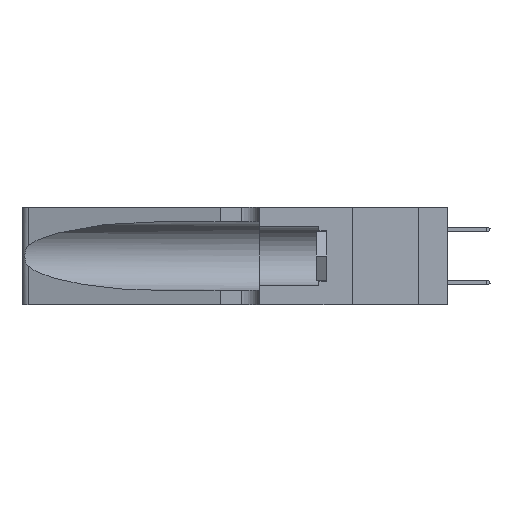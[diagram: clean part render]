
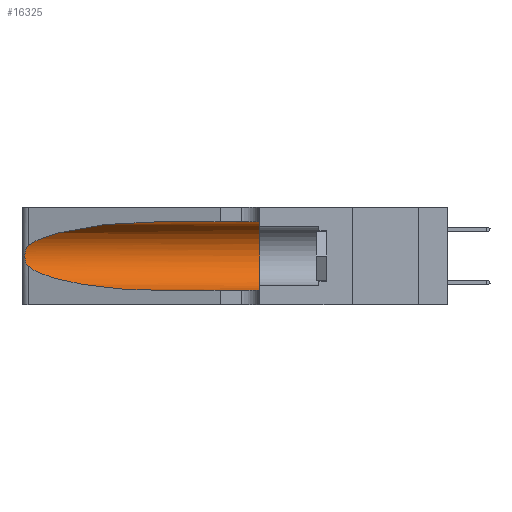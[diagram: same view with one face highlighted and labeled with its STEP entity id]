
A CAD part, left-side view. The second image highlights one B-rep face of the part: STEP entity #16325.
In plain terms, the highlighted cylindrical face has radius 3.308 mm (diameter 6.617 mm), a partial arc.
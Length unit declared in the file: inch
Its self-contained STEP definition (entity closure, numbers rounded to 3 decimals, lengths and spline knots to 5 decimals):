
#43 = CARTESIAN_POINT ( 'NONE',  ( 0.1305, 1.61858, 0.185 ) ) ;
#162 = ORIENTED_EDGE ( 'NONE', *, *, #4983, .F. ) ;
#1116 = CARTESIAN_POINT ( 'NONE',  ( 0.25487, 1.22718, 0.14631 ) ) ;
#1506 = CARTESIAN_POINT ( 'NONE',  ( 0.25555, 1.22994, 0.2215 ) ) ;
#3248 = B_SPLINE_CURVE_WITH_KNOTS ( 'NONE', 3,
 ( #15390, #1506, #21272, #32494, #4783, #7573, #10356, #21038, #30301, #34028, #19004, #22114, #27358, #10735 ),
 .UNSPECIFIED., .F., .F.,
 ( 4, 2, 2, 2, 2, 2, 4 ),
 ( 0., 0.00027, 0.00053, 0.00107, 0.0016, 0.00187, 0.00214 ),
 .UNSPECIFIED. ) ;
#3458 = ORIENTED_EDGE ( 'NONE', *, *, #6924, .T. ) ;
#4783 = CARTESIAN_POINT ( 'NONE',  ( 0.25854, 1.2359, 0.20912 ) ) ;
#4849 = ORIENTED_EDGE ( 'NONE', *, *, #20358, .T. ) ;
#4983 = EDGE_CURVE ( 'NONE', #24811, #6345, #30905, .T. ) ;
#5214 = VERTEX_POINT ( 'NONE', #15593 ) ;
#5854 = DIRECTION ( 'NONE',  ( 0., -1., 0. ) ) ;
#6345 = VERTEX_POINT ( 'NONE', #18593 ) ;
#6441 = VERTEX_POINT ( 'NONE', #10601 ) ;
#6924 = EDGE_CURVE ( 'NONE', #6441, #5214, #16180, .T. ) ;
#7409 = ORIENTED_EDGE ( 'NONE', *, *, #34758, .F. ) ;
#7573 = CARTESIAN_POINT ( 'NONE',  ( 0.26018, 1.23835, 0.19895 ) ) ;
#9037 = LINE ( 'NONE', #17661, #29029 ) ;
#10340 = CARTESIAN_POINT ( 'NONE',  ( 0.2373, 1.15595, 0.08982 ) ) ;
#10356 = CARTESIAN_POINT ( 'NONE',  ( 0.26075, 1.23896, 0.19203 ) ) ;
#10601 = CARTESIAN_POINT ( 'NONE',  ( 0.1305, 0.72297, 0.31525 ) ) ;
#10718 = CARTESIAN_POINT ( 'NONE',  ( 0.25487, 1.22718, 0.14631 ) ) ;
#10735 = CARTESIAN_POINT ( 'NONE',  ( 0.25487, 1.22718, 0.14631 ) ) ;
#11942 = DIRECTION ( 'NONE',  ( 0., -1., 0. ) ) ;
#13049 = CARTESIAN_POINT ( 'NONE',  ( 0.25487, 1.22718, 0.22369 ) ) ;
#13849 = CARTESIAN_POINT ( 'NONE',  ( 0.1305, 0.35, 0.185 ) ) ;
#15390 = CARTESIAN_POINT ( 'NONE',  ( 0.25487, 1.22718, 0.22369 ) ) ;
#15593 = CARTESIAN_POINT ( 'NONE',  ( 0.25487, 1.22718, 0.22369 ) ) ;
#15768 = CARTESIAN_POINT ( 'NONE',  ( 0.1305, 0.35, 0.31525 ) ) ;
#15977 = VERTEX_POINT ( 'NONE', #33857 ) ;
#15984 = FACE_OUTER_BOUND ( 'NONE', #34452, .T. ) ;
#16180 =( BOUNDED_CURVE ( )  B_SPLINE_CURVE ( 3, ( #24587, #35395, #29949, #13049 ),
 .UNSPECIFIED., .F., .F. ) 
 B_SPLINE_CURVE_WITH_KNOTS ( ( 4, 4 ),
 ( 1.5708, 2.84003 ),
 .UNSPECIFIED. ) 
 CURVE ( )  GEOMETRIC_REPRESENTATION_ITEM ( )  RATIONAL_B_SPLINE_CURVE ( ( 1., 0.87, 0.87, 1. ) ) 
 REPRESENTATION_ITEM ( '' )  );
#16193 = CARTESIAN_POINT ( 'NONE',  ( 0.18966, 0.96281, 0.05475 ) ) ;
#16325 = ADVANCED_FACE ( 'NONE', ( #15984 ), #25102, .F. ) ;
#16645 = DIRECTION ( 'NONE',  ( 0., 0., 1. ) ) ;
#17661 = CARTESIAN_POINT ( 'NONE',  ( 0.1305, 1.61858, 0.31525 ) ) ;
#18370 = EDGE_CURVE ( 'NONE', #5214, #28087, #3248, .T. ) ;
#18593 = CARTESIAN_POINT ( 'NONE',  ( 0.1305, 0.35, 0.05475 ) ) ;
#19004 = CARTESIAN_POINT ( 'NONE',  ( 0.25789, 1.23486, 0.15765 ) ) ;
#19466 = DIRECTION ( 'NONE',  ( 0., 0., -1. ) ) ;
#19686 = CARTESIAN_POINT ( 'NONE',  ( 0.1305, 1.61858, 0.05475 ) ) ;
#19943 =( BOUNDED_CURVE ( )  B_SPLINE_CURVE ( 3, ( #10718, #10340, #16193, #35750 ),
 .UNSPECIFIED., .F., .F. ) 
 B_SPLINE_CURVE_WITH_KNOTS ( ( 4, 4 ),
 ( 3.44316, 4.71239 ),
 .UNSPECIFIED. ) 
 CURVE ( )  GEOMETRIC_REPRESENTATION_ITEM ( )  RATIONAL_B_SPLINE_CURVE ( ( 1., 0.87, 0.87, 1. ) ) 
 REPRESENTATION_ITEM ( '' )  );
#20358 = EDGE_CURVE ( 'NONE', #15977, #6345, #30525, .T. ) ;
#21038 = CARTESIAN_POINT ( 'NONE',  ( 0.26075, 1.23896, 0.178 ) ) ;
#21272 = CARTESIAN_POINT ( 'NONE',  ( 0.25639, 1.23184, 0.21858 ) ) ;
#22114 = CARTESIAN_POINT ( 'NONE',  ( 0.25639, 1.23186, 0.15144 ) ) ;
#23569 = EDGE_CURVE ( 'NONE', #28087, #15977, #19943, .T. ) ;
#24587 = CARTESIAN_POINT ( 'NONE',  ( 0.1305, 0.72297, 0.31525 ) ) ;
#24811 = VERTEX_POINT ( 'NONE', #15768 ) ;
#25102 = CYLINDRICAL_SURFACE ( 'NONE', #32611, 0.13025 ) ;
#27358 = CARTESIAN_POINT ( 'NONE',  ( 0.25555, 1.22993, 0.14849 ) ) ;
#27604 = DIRECTION ( 'NONE',  ( 0., -1., 0. ) ) ;
#28087 = VERTEX_POINT ( 'NONE', #1116 ) ;
#29029 = VECTOR ( 'NONE', #11942, 39.37008 ) ;
#29114 = ORIENTED_EDGE ( 'NONE', *, *, #18370, .T. ) ;
#29949 = CARTESIAN_POINT ( 'NONE',  ( 0.2373, 1.15595, 0.28018 ) ) ;
#30301 = CARTESIAN_POINT ( 'NONE',  ( 0.26017, 1.23833, 0.17102 ) ) ;
#30525 = LINE ( 'NONE', #19686, #35251 ) ;
#30905 = CIRCLE ( 'NONE', #32600, 0.13025 ) ;
#32494 = CARTESIAN_POINT ( 'NONE',  ( 0.25787, 1.23484, 0.2124 ) ) ;
#32600 = AXIS2_PLACEMENT_3D ( 'NONE', #13849, #33290, #16645 ) ;
#32611 = AXIS2_PLACEMENT_3D ( 'NONE', #43, #27604, #19466 ) ;
#33290 = DIRECTION ( 'NONE',  ( 0., 1., 0. ) ) ;
#33857 = CARTESIAN_POINT ( 'NONE',  ( 0.1305, 0.72297, 0.05475 ) ) ;
#34028 = CARTESIAN_POINT ( 'NONE',  ( 0.25856, 1.23593, 0.16098 ) ) ;
#34452 = EDGE_LOOP ( 'NONE', ( #3458, #29114, #35661, #4849, #162, #7409 ) ) ;
#34758 = EDGE_CURVE ( 'NONE', #6441, #24811, #9037, .T. ) ;
#35251 = VECTOR ( 'NONE', #5854, 39.37008 ) ;
#35395 = CARTESIAN_POINT ( 'NONE',  ( 0.18966, 0.96281, 0.31525 ) ) ;
#35661 = ORIENTED_EDGE ( 'NONE', *, *, #23569, .T. ) ;
#35750 = CARTESIAN_POINT ( 'NONE',  ( 0.1305, 0.72297, 0.05475 ) ) ;
